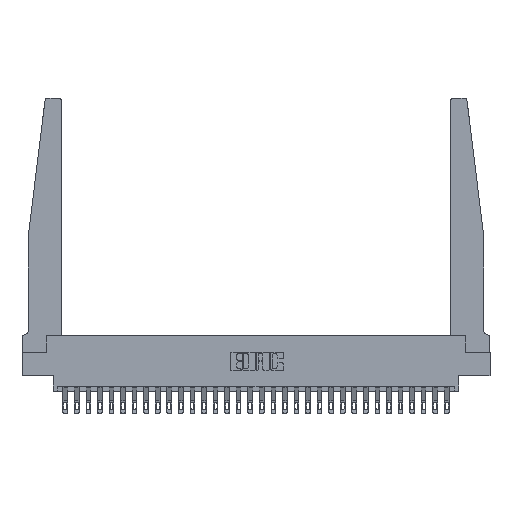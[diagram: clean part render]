
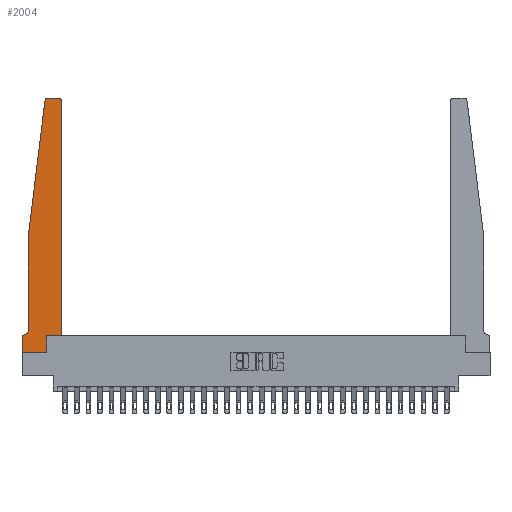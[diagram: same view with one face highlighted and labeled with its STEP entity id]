
A CAD part, top view. The second image highlights one B-rep face of the part: STEP entity #2004.
In plain terms, the highlighted planar face has unit normal (0, 0, 1).
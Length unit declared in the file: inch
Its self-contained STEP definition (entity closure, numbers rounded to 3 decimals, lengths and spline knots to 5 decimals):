
#35 = ORIENTED_EDGE ( 'NONE', *, *, #20718, .T. ) ;
#101 = DIRECTION ( 'NONE',  ( 0., 1., 0. ) ) ;
#170 = EDGE_CURVE ( 'NONE', #1648, #21060, #1452, .T. ) ;
#270 = VERTEX_POINT ( 'NONE', #23573 ) ;
#862 = CARTESIAN_POINT ( 'NONE',  ( 0.425, 0.18, 0.37 ) ) ;
#1452 = LINE ( 'NONE', #10073, #7313 ) ;
#1648 = VERTEX_POINT ( 'NONE', #24665 ) ;
#1697 = ORIENTED_EDGE ( 'NONE', *, *, #8623, .T. ) ;
#1796 = CARTESIAN_POINT ( 'NONE',  ( 0.065, 0.2375, 0.37 ) ) ;
#2004 = ADVANCED_FACE ( 'NONE', ( #3413 ), #22587, .T. ) ;
#3269 = EDGE_CURVE ( 'NONE', #21060, #270, #13368, .T. ) ;
#3383 = CARTESIAN_POINT ( 'NONE',  ( 0.24675, 2.72367, 0.37 ) ) ;
#3413 = FACE_OUTER_BOUND ( 'NONE', #11172, .T. ) ;
#3788 = DIRECTION ( 'NONE',  ( 0., -1., 0. ) ) ;
#3825 = EDGE_CURVE ( 'NONE', #10645, #1648, #5757, .T. ) ;
#3980 = VECTOR ( 'NONE', #18778, 39.37008 ) ;
#4401 = CARTESIAN_POINT ( 'NONE',  ( 0.395, 2.72, 0.37 ) ) ;
#4713 = ORIENTED_EDGE ( 'NONE', *, *, #3825, .T. ) ;
#5463 = ORIENTED_EDGE ( 'NONE', *, *, #21962, .T. ) ;
#5757 = LINE ( 'NONE', #12880, #22655 ) ;
#5830 = AXIS2_PLACEMENT_3D ( 'NONE', #18186, #9398, #24811 ) ;
#6020 = LINE ( 'NONE', #862, #17102 ) ;
#6119 = LINE ( 'NONE', #12595, #11310 ) ;
#6607 = DIRECTION ( 'NONE',  ( 1., 0., 0. ) ) ;
#6740 = ORIENTED_EDGE ( 'NONE', *, *, #15279, .T. ) ;
#7313 = VECTOR ( 'NONE', #25507, 39.37008 ) ;
#7359 = LINE ( 'NONE', #28169, #18413 ) ;
#7482 = VECTOR ( 'NONE', #101, 39.37008 ) ;
#7967 = VERTEX_POINT ( 'NONE', #26634 ) ;
#8255 = CARTESIAN_POINT ( 'NONE',  ( 0., 0.1875, 0.37 ) ) ;
#8598 = CARTESIAN_POINT ( 'NONE',  ( 0.065, 0.1875, 0.37 ) ) ;
#8623 = EDGE_CURVE ( 'NONE', #18722, #28205, #13547, .T. ) ;
#8660 = AXIS2_PLACEMENT_3D ( 'NONE', #12395, #27773, #14608 ) ;
#8845 = CARTESIAN_POINT ( 'NONE',  ( 0.2605, 0.18, 0.37 ) ) ;
#9398 = DIRECTION ( 'NONE',  ( 0., 0., 1. ) ) ;
#9575 = VERTEX_POINT ( 'NONE', #19361 ) ;
#9835 = AXIS2_PLACEMENT_3D ( 'NONE', #12296, #27685, #14527 ) ;
#10073 = CARTESIAN_POINT ( 'NONE',  ( 0., 0., 0.37 ) ) ;
#10645 = VERTEX_POINT ( 'NONE', #8255 ) ;
#10821 = DIRECTION ( 'NONE',  ( -1., 0., 0. ) ) ;
#11036 = EDGE_CURVE ( 'NONE', #16259, #9575, #26480, .T. ) ;
#11172 = EDGE_LOOP ( 'NONE', ( #21118, #6740, #1697, #23549, #16605, #35, #4713, #24519, #16407, #14818, #17735, #5463 ) ) ;
#11310 = VECTOR ( 'NONE', #23270, 39.37008 ) ;
#12223 = VERTEX_POINT ( 'NONE', #27615 ) ;
#12296 = CARTESIAN_POINT ( 'NONE',  ( 0.27653, 2.72, 0.37 ) ) ;
#12395 = CARTESIAN_POINT ( 'NONE',  ( 0.015, 0.2375, 0.37 ) ) ;
#12595 = CARTESIAN_POINT ( 'NONE',  ( 0.425, 0.18, 0.37 ) ) ;
#12880 = CARTESIAN_POINT ( 'NONE',  ( 0., 0., 0.37 ) ) ;
#13368 = LINE ( 'NONE', #8845, #7482 ) ;
#13377 = CARTESIAN_POINT ( 'NONE',  ( 0.065, 1.25, 0.37 ) ) ;
#13451 = EDGE_CURVE ( 'NONE', #28409, #12223, #21567, .T. ) ;
#13547 = LINE ( 'NONE', #26785, #24563 ) ;
#14349 = LINE ( 'NONE', #8598, #24678 ) ;
#14527 = DIRECTION ( 'NONE',  ( 1., 0., 0. ) ) ;
#14608 = DIRECTION ( 'NONE',  ( -1., 0., 0. ) ) ;
#14818 = ORIENTED_EDGE ( 'NONE', *, *, #26026, .T. ) ;
#15279 = EDGE_CURVE ( 'NONE', #12223, #18722, #23610, .T. ) ;
#15850 = DIRECTION ( 'NONE',  ( -0.122, -0.992, 0. ) ) ;
#16250 = EDGE_CURVE ( 'NONE', #28205, #16259, #7359, .T. ) ;
#16259 = VERTEX_POINT ( 'NONE', #1796 ) ;
#16407 = ORIENTED_EDGE ( 'NONE', *, *, #3269, .T. ) ;
#16576 = CARTESIAN_POINT ( 'NONE',  ( 0.25, 2.75, 0.37 ) ) ;
#16605 = ORIENTED_EDGE ( 'NONE', *, *, #11036, .T. ) ;
#17102 = VECTOR ( 'NONE', #20692, 39.37008 ) ;
#17345 = VERTEX_POINT ( 'NONE', #18888 ) ;
#17735 = ORIENTED_EDGE ( 'NONE', *, *, #21573, .T. ) ;
#18186 = CARTESIAN_POINT ( 'NONE',  ( 0., 0.1875, 0.37 ) ) ;
#18413 = VECTOR ( 'NONE', #3788, 39.37008 ) ;
#18533 = CARTESIAN_POINT ( 'NONE',  ( 0.2605, 0., 0.37 ) ) ;
#18722 = VERTEX_POINT ( 'NONE', #3383 ) ;
#18778 = DIRECTION ( 'NONE',  ( -1., 0., 0. ) ) ;
#18888 = CARTESIAN_POINT ( 'NONE',  ( 0.425, 0.18, 0.37 ) ) ;
#19361 = CARTESIAN_POINT ( 'NONE',  ( 0.015, 0.1875, 0.37 ) ) ;
#19825 = DIRECTION ( 'NONE',  ( 0., 0., 1. ) ) ;
#20692 = DIRECTION ( 'NONE',  ( 0., 1., 0. ) ) ;
#20718 = EDGE_CURVE ( 'NONE', #9575, #10645, #14349, .T. ) ;
#21060 = VERTEX_POINT ( 'NONE', #18533 ) ;
#21118 = ORIENTED_EDGE ( 'NONE', *, *, #13451, .T. ) ;
#21567 = LINE ( 'NONE', #16576, #3980 ) ;
#21573 = EDGE_CURVE ( 'NONE', #17345, #7967, #6020, .T. ) ;
#21962 = EDGE_CURVE ( 'NONE', #7967, #28409, #24976, .T. ) ;
#22587 = PLANE ( 'NONE',  #5830 ) ;
#22655 = VECTOR ( 'NONE', #28379, 39.37008 ) ;
#23270 = DIRECTION ( 'NONE',  ( 1., 0., 0. ) ) ;
#23352 = CARTESIAN_POINT ( 'NONE',  ( 0.395, 2.75, 0.37 ) ) ;
#23549 = ORIENTED_EDGE ( 'NONE', *, *, #16250, .T. ) ;
#23573 = CARTESIAN_POINT ( 'NONE',  ( 0.2605, 0.18, 0.37 ) ) ;
#23610 = CIRCLE ( 'NONE', #9835, 0.03 ) ;
#24519 = ORIENTED_EDGE ( 'NONE', *, *, #170, .T. ) ;
#24563 = VECTOR ( 'NONE', #15850, 39.37008 ) ;
#24665 = CARTESIAN_POINT ( 'NONE',  ( 0., 0., 0.37 ) ) ;
#24678 = VECTOR ( 'NONE', #10821, 39.37008 ) ;
#24811 = DIRECTION ( 'NONE',  ( 1., 0., 0. ) ) ;
#24976 = CIRCLE ( 'NONE', #25999, 0.03 ) ;
#25507 = DIRECTION ( 'NONE',  ( 1., 0., 0. ) ) ;
#25999 = AXIS2_PLACEMENT_3D ( 'NONE', #4401, #19825, #6607 ) ;
#26026 = EDGE_CURVE ( 'NONE', #270, #17345, #6119, .T. ) ;
#26480 = CIRCLE ( 'NONE', #8660, 0.05 ) ;
#26634 = CARTESIAN_POINT ( 'NONE',  ( 0.425, 2.72, 0.37 ) ) ;
#26785 = CARTESIAN_POINT ( 'NONE',  ( 0.065, 1.25, 0.37 ) ) ;
#27615 = CARTESIAN_POINT ( 'NONE',  ( 0.27653, 2.75, 0.37 ) ) ;
#27685 = DIRECTION ( 'NONE',  ( 0., 0., 1. ) ) ;
#27773 = DIRECTION ( 'NONE',  ( 0., 0., -1. ) ) ;
#28169 = CARTESIAN_POINT ( 'NONE',  ( 0.065, 1.25, 0.37 ) ) ;
#28205 = VERTEX_POINT ( 'NONE', #13377 ) ;
#28379 = DIRECTION ( 'NONE',  ( 0., -1., 0. ) ) ;
#28409 = VERTEX_POINT ( 'NONE', #23352 ) ;
